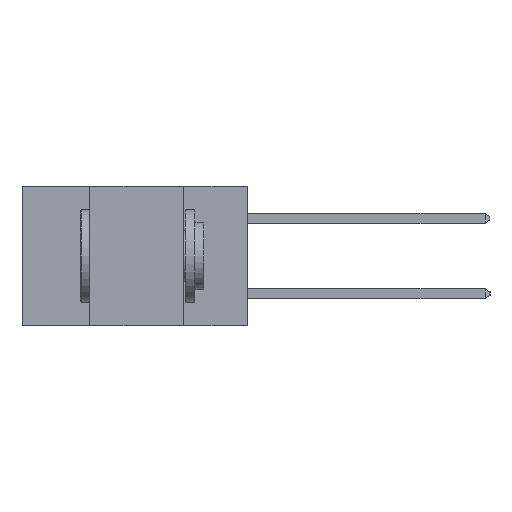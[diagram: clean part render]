
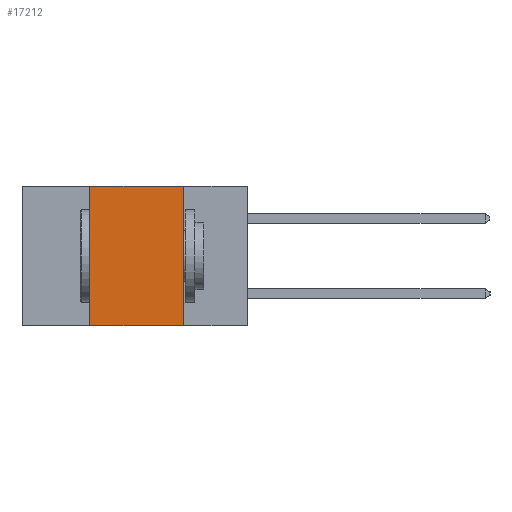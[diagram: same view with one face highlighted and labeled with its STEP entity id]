
A CAD part, left-side view. The second image highlights one B-rep face of the part: STEP entity #17212.
In plain terms, the highlighted planar face has unit normal (-1, 0, 0).
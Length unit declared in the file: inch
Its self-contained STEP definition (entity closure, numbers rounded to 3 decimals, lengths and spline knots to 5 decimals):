
#243 = DIRECTION ( 'NONE',  ( 0., 0., 1. ) ) ;
#247 = ORIENTED_EDGE ( 'NONE', *, *, #10373, .F. ) ;
#1048 = ORIENTED_EDGE ( 'NONE', *, *, #6454, .T. ) ;
#1077 = VERTEX_POINT ( 'NONE', #11776 ) ;
#1920 = VECTOR ( 'NONE', #243, 39.37008 ) ;
#2797 = VERTEX_POINT ( 'NONE', #12976 ) ;
#3178 = ORIENTED_EDGE ( 'NONE', *, *, #7428, .F. ) ;
#3755 = CARTESIAN_POINT ( 'NONE',  ( 0., 0.6, 0. ) ) ;
#4800 = DIRECTION ( 'NONE',  ( 0., 0., -1. ) ) ;
#5449 = CARTESIAN_POINT ( 'NONE',  ( 0., 0.6, -0.37 ) ) ;
#5562 = VERTEX_POINT ( 'NONE', #7718 ) ;
#5829 = LINE ( 'NONE', #17497, #1920 ) ;
#6454 = EDGE_CURVE ( 'NONE', #14643, #2797, #14928, .T. ) ;
#7139 = CARTESIAN_POINT ( 'NONE',  ( 0., 0.42, -0.37 ) ) ;
#7428 = EDGE_CURVE ( 'NONE', #14643, #5562, #5829, .T. ) ;
#7718 = CARTESIAN_POINT ( 'NONE',  ( 0., 0.42, 0. ) ) ;
#7914 = CARTESIAN_POINT ( 'NONE',  ( 0., 0.6, 0. ) ) ;
#7976 = DIRECTION ( 'NONE',  ( 1., 0., 0. ) ) ;
#8397 = EDGE_CURVE ( 'NONE', #5562, #1077, #9260, .T. ) ;
#8786 = VECTOR ( 'NONE', #13935, 39.37008 ) ;
#9260 = LINE ( 'NONE', #3755, #8786 ) ;
#10373 = EDGE_CURVE ( 'NONE', #1077, #2797, #17486, .T. ) ;
#11776 = CARTESIAN_POINT ( 'NONE',  ( 0., 0.17, 0. ) ) ;
#11951 = EDGE_LOOP ( 'NONE', ( #247, #18440, #3178, #1048 ) ) ;
#12976 = CARTESIAN_POINT ( 'NONE',  ( 0., 0.17, -0.37 ) ) ;
#13022 = AXIS2_PLACEMENT_3D ( 'NONE', #7914, #7976, #17922 ) ;
#13735 = PLANE ( 'NONE',  #13022 ) ;
#13935 = DIRECTION ( 'NONE',  ( 0., -1., 0. ) ) ;
#14643 = VERTEX_POINT ( 'NONE', #7139 ) ;
#14928 = LINE ( 'NONE', #5449, #18576 ) ;
#15488 = FACE_OUTER_BOUND ( 'NONE', #11951, .T. ) ;
#15558 = DIRECTION ( 'NONE',  ( 0., -1., 0. ) ) ;
#17042 = VECTOR ( 'NONE', #4800, 39.37008 ) ;
#17212 = ADVANCED_FACE ( 'NONE', ( #15488 ), #13735, .F. ) ;
#17486 = LINE ( 'NONE', #17633, #17042 ) ;
#17497 = CARTESIAN_POINT ( 'NONE',  ( 0., 0.42, -0.37 ) ) ;
#17633 = CARTESIAN_POINT ( 'NONE',  ( 0., 0.17, -0.37 ) ) ;
#17922 = DIRECTION ( 'NONE',  ( 0., 0., -1. ) ) ;
#18440 = ORIENTED_EDGE ( 'NONE', *, *, #8397, .F. ) ;
#18576 = VECTOR ( 'NONE', #15558, 39.37008 ) ;
